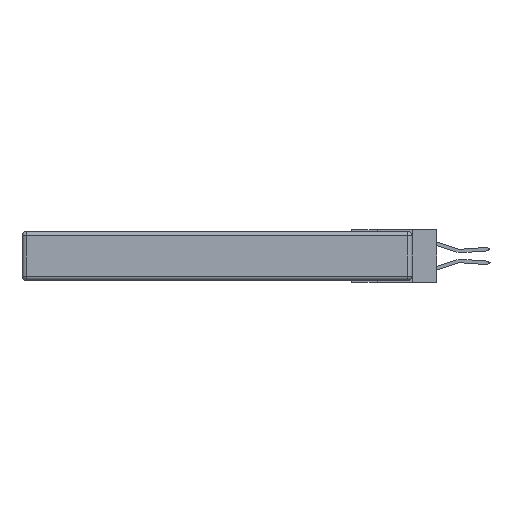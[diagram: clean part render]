
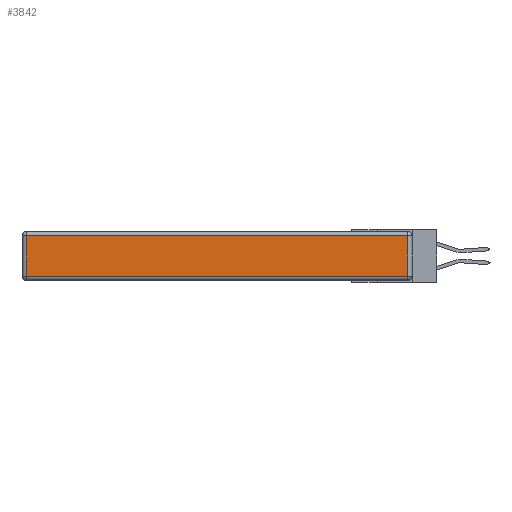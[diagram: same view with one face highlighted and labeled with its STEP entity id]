
A CAD part, left-side view. The second image highlights one B-rep face of the part: STEP entity #3842.
In plain terms, the highlighted planar face has unit normal (-1, 0, 0).
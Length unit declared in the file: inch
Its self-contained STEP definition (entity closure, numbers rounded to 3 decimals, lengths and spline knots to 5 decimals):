
#129 = LINE ( 'NONE', #4896, #10501 ) ;
#195 = LINE ( 'NONE', #11918, #6031 ) ;
#1163 = LINE ( 'NONE', #9771, #6416 ) ;
#1373 = ORIENTED_EDGE ( 'NONE', *, *, #5293, .T. ) ;
#1608 = VERTEX_POINT ( 'NONE', #14091 ) ;
#2165 = CARTESIAN_POINT ( 'NONE',  ( 0., 2.72, -0.03 ) ) ;
#2621 = EDGE_LOOP ( 'NONE', ( #12921, #10626, #14920, #1373 ) ) ;
#2979 = CARTESIAN_POINT ( 'NONE',  ( 0., 0.03, -0.03 ) ) ;
#3155 = CARTESIAN_POINT ( 'NONE',  ( 0., 0., -0.343 ) ) ;
#3842 = ADVANCED_FACE ( 'NONE', ( #10604 ), #10395, .T. ) ;
#3894 = DIRECTION ( 'NONE',  ( 0., 1., 0. ) ) ;
#4215 = VERTEX_POINT ( 'NONE', #15063 ) ;
#4364 = DIRECTION ( 'NONE',  ( 0., 0., 1. ) ) ;
#4896 = CARTESIAN_POINT ( 'NONE',  ( 0., 2.75, -0.03 ) ) ;
#5095 = DIRECTION ( 'NONE',  ( 0., 0., 1. ) ) ;
#5293 = EDGE_CURVE ( 'NONE', #7849, #1608, #195, .T. ) ;
#5723 = LINE ( 'NONE', #12469, #13252 ) ;
#6031 = VECTOR ( 'NONE', #8359, 39.37008 ) ;
#6416 = VECTOR ( 'NONE', #5095, 39.37008 ) ;
#7085 = AXIS2_PLACEMENT_3D ( 'NONE', #3155, #11639, #4364 ) ;
#7276 = EDGE_CURVE ( 'NONE', #13267, #7849, #129, .T. ) ;
#7849 = VERTEX_POINT ( 'NONE', #2165 ) ;
#8359 = DIRECTION ( 'NONE',  ( 0., 0., -1. ) ) ;
#8542 = EDGE_CURVE ( 'NONE', #1608, #4215, #5723, .T. ) ;
#9771 = CARTESIAN_POINT ( 'NONE',  ( 0., 0.03, -0.343 ) ) ;
#10395 = PLANE ( 'NONE',  #7085 ) ;
#10501 = VECTOR ( 'NONE', #3894, 39.37008 ) ;
#10604 = FACE_OUTER_BOUND ( 'NONE', #2621, .T. ) ;
#10626 = ORIENTED_EDGE ( 'NONE', *, *, #12461, .T. ) ;
#11435 = DIRECTION ( 'NONE',  ( 0., -1., 0. ) ) ;
#11639 = DIRECTION ( 'NONE',  ( -1., 0., 0. ) ) ;
#11918 = CARTESIAN_POINT ( 'NONE',  ( 0., 2.72, -0.343 ) ) ;
#12461 = EDGE_CURVE ( 'NONE', #4215, #13267, #1163, .T. ) ;
#12469 = CARTESIAN_POINT ( 'NONE',  ( 0., 0., -0.313 ) ) ;
#12921 = ORIENTED_EDGE ( 'NONE', *, *, #8542, .T. ) ;
#13252 = VECTOR ( 'NONE', #11435, 39.37008 ) ;
#13267 = VERTEX_POINT ( 'NONE', #2979 ) ;
#14091 = CARTESIAN_POINT ( 'NONE',  ( 0., 2.72, -0.313 ) ) ;
#14920 = ORIENTED_EDGE ( 'NONE', *, *, #7276, .T. ) ;
#15063 = CARTESIAN_POINT ( 'NONE',  ( 0., 0.03, -0.313 ) ) ;
